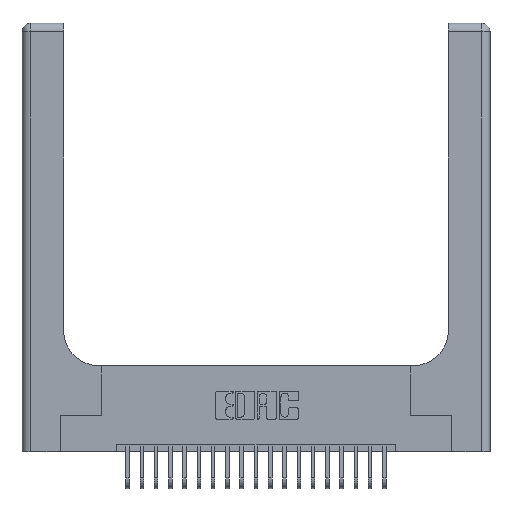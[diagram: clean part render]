
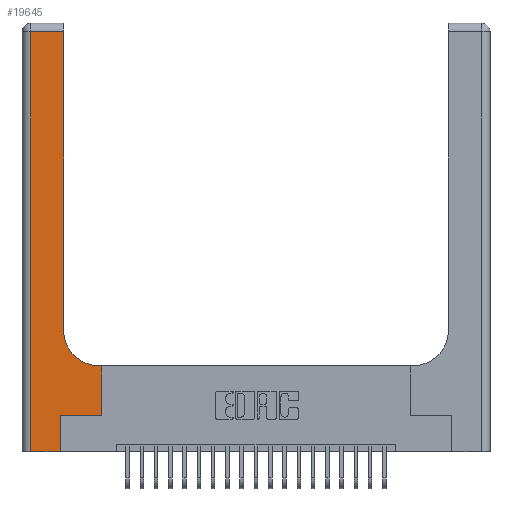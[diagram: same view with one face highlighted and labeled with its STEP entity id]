
A CAD part, top view. The second image highlights one B-rep face of the part: STEP entity #19645.
In plain terms, the highlighted planar face has unit normal (0, 0, 1).
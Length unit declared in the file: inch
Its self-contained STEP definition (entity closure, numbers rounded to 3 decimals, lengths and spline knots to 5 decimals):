
#643 = LINE ( 'NONE', #9035, #14848 ) ;
#818 = DIRECTION ( 'NONE',  ( -1., 0., 0. ) ) ;
#1261 = CARTESIAN_POINT ( 'NONE',  ( 0.5585, 0.25, 0.37 ) ) ;
#1834 = CARTESIAN_POINT ( 'NONE',  ( 0.2915, 0.85, 0.37 ) ) ;
#2071 = DIRECTION ( 'NONE',  ( -1., 0., 0. ) ) ;
#2284 = ORIENTED_EDGE ( 'NONE', *, *, #4489, .T. ) ;
#2569 = VECTOR ( 'NONE', #8566, 39.37008 ) ;
#3036 = ORIENTED_EDGE ( 'NONE', *, *, #23085, .T. ) ;
#3245 = DIRECTION ( 'NONE',  ( 0., 1., 0. ) ) ;
#3326 = DIRECTION ( 'NONE',  ( 0., 0., -1. ) ) ;
#3345 = VECTOR ( 'NONE', #16819, 39.37008 ) ;
#3601 = ORIENTED_EDGE ( 'NONE', *, *, #12164, .T. ) ;
#4489 = EDGE_CURVE ( 'NONE', #10964, #9122, #643, .T. ) ;
#4975 = LINE ( 'NONE', #7821, #8275 ) ;
#6067 = LINE ( 'NONE', #13512, #11194 ) ;
#6234 = CARTESIAN_POINT ( 'NONE',  ( 0.5415, 0.85, 0.37 ) ) ;
#6249 = CARTESIAN_POINT ( 'NONE',  ( 0.5415, 0.6, 0.37 ) ) ;
#6373 = CARTESIAN_POINT ( 'NONE',  ( 0.2915, 2.94, 0.37 ) ) ;
#7070 = EDGE_CURVE ( 'NONE', #8521, #16591, #21307, .T. ) ;
#7168 = CARTESIAN_POINT ( 'NONE',  ( 0., 0., 0.37 ) ) ;
#7735 = LINE ( 'NONE', #18158, #2569 ) ;
#7821 = CARTESIAN_POINT ( 'NONE',  ( 0., 2.94, 0.37 ) ) ;
#8159 = DIRECTION ( 'NONE',  ( 1., 0., 0. ) ) ;
#8275 = VECTOR ( 'NONE', #2071, 39.37008 ) ;
#8495 = EDGE_CURVE ( 'NONE', #18004, #8521, #13594, .T. ) ;
#8521 = VERTEX_POINT ( 'NONE', #13264 ) ;
#8566 = DIRECTION ( 'NONE',  ( 0., 1., 0. ) ) ;
#8604 = EDGE_CURVE ( 'NONE', #22142, #11379, #6067, .T. ) ;
#9035 = CARTESIAN_POINT ( 'NONE',  ( 0.06, 3., 0.37 ) ) ;
#9122 = VERTEX_POINT ( 'NONE', #17194 ) ;
#9668 = EDGE_CURVE ( 'NONE', #9122, #22750, #13571, .T. ) ;
#9924 = ORIENTED_EDGE ( 'NONE', *, *, #8495, .T. ) ;
#10212 = ORIENTED_EDGE ( 'NONE', *, *, #20590, .T. ) ;
#10750 = ORIENTED_EDGE ( 'NONE', *, *, #14990, .T. ) ;
#10945 = CARTESIAN_POINT ( 'NONE',  ( 0.06, 2.94, 0.37 ) ) ;
#10964 = VERTEX_POINT ( 'NONE', #10945 ) ;
#11127 = VECTOR ( 'NONE', #3245, 39.37008 ) ;
#11194 = VECTOR ( 'NONE', #13674, 39.37008 ) ;
#11379 = VERTEX_POINT ( 'NONE', #6373 ) ;
#12164 = EDGE_CURVE ( 'NONE', #16591, #14459, #13453, .T. ) ;
#12825 = DIRECTION ( 'NONE',  ( 0., -1., 0. ) ) ;
#13264 = CARTESIAN_POINT ( 'NONE',  ( 0.5585, 0.25, 0.37 ) ) ;
#13453 = LINE ( 'NONE', #14321, #17967 ) ;
#13512 = CARTESIAN_POINT ( 'NONE',  ( 0.2915, 3., 0.37 ) ) ;
#13571 = LINE ( 'NONE', #7168, #3345 ) ;
#13594 = LINE ( 'NONE', #17047, #23138 ) ;
#13674 = DIRECTION ( 'NONE',  ( 0., 1., 0. ) ) ;
#14321 = CARTESIAN_POINT ( 'NONE',  ( 0.2915, 0.6, 0.37 ) ) ;
#14459 = VERTEX_POINT ( 'NONE', #6249 ) ;
#14462 = CIRCLE ( 'NONE', #19151, 0.25 ) ;
#14651 = ORIENTED_EDGE ( 'NONE', *, *, #8604, .T. ) ;
#14846 = CARTESIAN_POINT ( 'NONE',  ( 0., 3., 0.37 ) ) ;
#14848 = VECTOR ( 'NONE', #12825, 39.37008 ) ;
#14925 = AXIS2_PLACEMENT_3D ( 'NONE', #14846, #3326, #16763 ) ;
#14990 = EDGE_CURVE ( 'NONE', #11379, #10964, #4975, .T. ) ;
#15558 = ORIENTED_EDGE ( 'NONE', *, *, #9668, .T. ) ;
#16591 = VERTEX_POINT ( 'NONE', #20519 ) ;
#16742 = ORIENTED_EDGE ( 'NONE', *, *, #7070, .T. ) ;
#16763 = DIRECTION ( 'NONE',  ( -1., 0., 0. ) ) ;
#16790 = FACE_OUTER_BOUND ( 'NONE', #21925, .T. ) ;
#16819 = DIRECTION ( 'NONE',  ( 1., 0., 0. ) ) ;
#17047 = CARTESIAN_POINT ( 'NONE',  ( 0.269, 0.25, 0.37 ) ) ;
#17194 = CARTESIAN_POINT ( 'NONE',  ( 0.06, 0., 0.37 ) ) ;
#17967 = VECTOR ( 'NONE', #818, 39.37008 ) ;
#18004 = VERTEX_POINT ( 'NONE', #20567 ) ;
#18158 = CARTESIAN_POINT ( 'NONE',  ( 0.269, 0., 0.37 ) ) ;
#18429 = CARTESIAN_POINT ( 'NONE',  ( 0.269, 0., 0.37 ) ) ;
#18982 = DIRECTION ( 'NONE',  ( 1., 0., 0. ) ) ;
#19151 = AXIS2_PLACEMENT_3D ( 'NONE', #6234, #19667, #8159 ) ;
#19645 = ADVANCED_FACE ( 'NONE', ( #16790 ), #20549, .F. ) ;
#19667 = DIRECTION ( 'NONE',  ( 0., 0., -1. ) ) ;
#20519 = CARTESIAN_POINT ( 'NONE',  ( 0.5585, 0.6, 0.37 ) ) ;
#20549 = PLANE ( 'NONE',  #14925 ) ;
#20567 = CARTESIAN_POINT ( 'NONE',  ( 0.269, 0.25, 0.37 ) ) ;
#20590 = EDGE_CURVE ( 'NONE', #22750, #18004, #7735, .T. ) ;
#21307 = LINE ( 'NONE', #1261, #11127 ) ;
#21925 = EDGE_LOOP ( 'NONE', ( #14651, #10750, #2284, #15558, #10212, #9924, #16742, #3601, #3036 ) ) ;
#22142 = VERTEX_POINT ( 'NONE', #1834 ) ;
#22750 = VERTEX_POINT ( 'NONE', #18429 ) ;
#23085 = EDGE_CURVE ( 'NONE', #14459, #22142, #14462, .T. ) ;
#23138 = VECTOR ( 'NONE', #18982, 39.37008 ) ;
